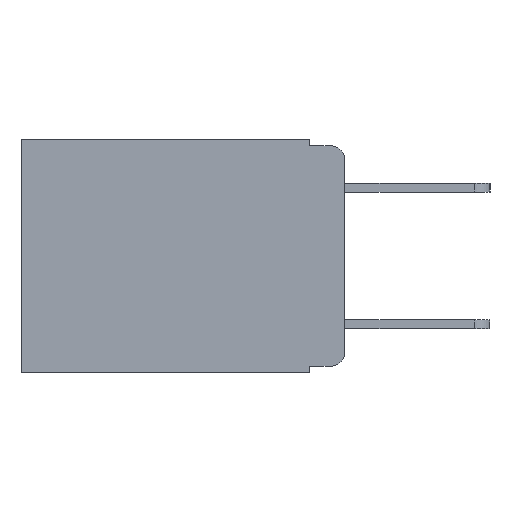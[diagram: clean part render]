
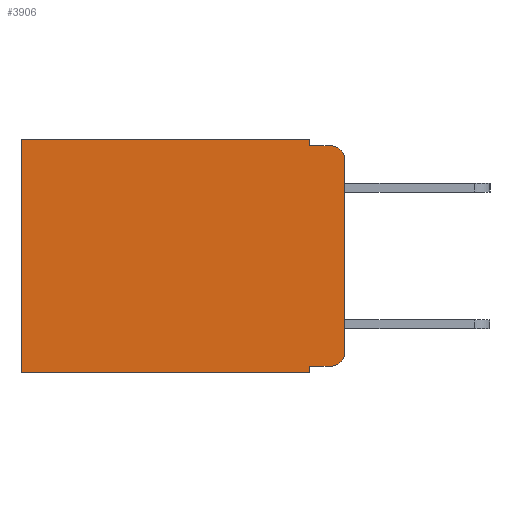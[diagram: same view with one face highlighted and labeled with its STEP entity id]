
A CAD part, left-side view. The second image highlights one B-rep face of the part: STEP entity #3906.
In plain terms, the highlighted planar face has unit normal (-1, 0, 0).
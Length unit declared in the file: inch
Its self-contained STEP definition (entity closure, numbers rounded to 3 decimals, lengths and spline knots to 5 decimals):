
#82 = CARTESIAN_POINT ( 'NONE',  ( 0.298, 0., -0.343 ) ) ;
#286 = CARTESIAN_POINT ( 'NONE',  ( 0.298, 0., 0. ) ) ;
#408 = AXIS2_PLACEMENT_3D ( 'NONE', #286, #2513, #8446 ) ;
#623 = CIRCLE ( 'NONE', #1907, 0.02 ) ;
#673 = LINE ( 'NONE', #2784, #7673 ) ;
#875 = CARTESIAN_POINT ( 'NONE',  ( 0.298, 0., 0. ) ) ;
#1018 = CARTESIAN_POINT ( 'NONE',  ( 0.298, 0., -0.313 ) ) ;
#1163 = LINE ( 'NONE', #875, #3454 ) ;
#1199 = EDGE_LOOP ( 'NONE', ( #7151, #10430, #8244, #7277, #4624, #6740, #10319, #8763, #6346, #9999 ) ) ;
#1327 = CARTESIAN_POINT ( 'NONE',  ( 0.298, 0., -0.03 ) ) ;
#1535 = VERTEX_POINT ( 'NONE', #8082 ) ;
#1851 = LINE ( 'NONE', #7398, #3890 ) ;
#1907 = AXIS2_PLACEMENT_3D ( 'NONE', #8008, #7997, #8992 ) ;
#2080 = CARTESIAN_POINT ( 'NONE',  ( 0.298, 0.051, -0.333 ) ) ;
#2082 = DIRECTION ( 'NONE',  ( 0., 0., -1. ) ) ;
#2168 = VERTEX_POINT ( 'NONE', #8883 ) ;
#2513 = DIRECTION ( 'NONE',  ( 1., 0., 0. ) ) ;
#2743 = CARTESIAN_POINT ( 'NONE',  ( 0.298, 0.02, -0.01 ) ) ;
#2784 = CARTESIAN_POINT ( 'NONE',  ( 0.298, 0.473, 0. ) ) ;
#2931 = VECTOR ( 'NONE', #10050, 39.37008 ) ;
#3118 = DIRECTION ( 'NONE',  ( 0., 0., -1. ) ) ;
#3124 = CARTESIAN_POINT ( 'NONE',  ( 0.298, 0.051, 0. ) ) ;
#3155 = CARTESIAN_POINT ( 'NONE',  ( 0.298, 0.051, 0. ) ) ;
#3364 = EDGE_CURVE ( 'NONE', #9633, #1535, #4097, .T. ) ;
#3365 = CIRCLE ( 'NONE', #4698, 0.02 ) ;
#3454 = VECTOR ( 'NONE', #5291, 39.37008 ) ;
#3890 = VECTOR ( 'NONE', #7408, 39.37008 ) ;
#3906 = ADVANCED_FACE ( 'NONE', ( #4807 ), #8005, .F. ) ;
#3939 = CARTESIAN_POINT ( 'NONE',  ( 0.298, 0.473, 0. ) ) ;
#3968 = VERTEX_POINT ( 'NONE', #2743 ) ;
#4042 = VERTEX_POINT ( 'NONE', #3124 ) ;
#4097 = LINE ( 'NONE', #82, #6246 ) ;
#4111 = DIRECTION ( 'NONE',  ( 0., 0., -1. ) ) ;
#4211 = DIRECTION ( 'NONE',  ( 0., 0., -1. ) ) ;
#4363 = EDGE_CURVE ( 'NONE', #5120, #5538, #3365, .T. ) ;
#4473 = EDGE_CURVE ( 'NONE', #2168, #5120, #8553, .T. ) ;
#4617 = EDGE_CURVE ( 'NONE', #2168, #9633, #9117, .T. ) ;
#4624 = ORIENTED_EDGE ( 'NONE', *, *, #6464, .T. ) ;
#4626 = DIRECTION ( 'NONE',  ( 0., 1., 0. ) ) ;
#4658 = CARTESIAN_POINT ( 'NONE',  ( 0.298, 0.051, -0.01 ) ) ;
#4698 = AXIS2_PLACEMENT_3D ( 'NONE', #10619, #10212, #4111 ) ;
#4703 = EDGE_CURVE ( 'NONE', #6406, #1535, #673, .T. ) ;
#4765 = DIRECTION ( 'NONE',  ( 0., -1., 0. ) ) ;
#4787 = EDGE_CURVE ( 'NONE', #4042, #5731, #10250, .T. ) ;
#4807 = FACE_OUTER_BOUND ( 'NONE', #1199, .T. ) ;
#5120 = VERTEX_POINT ( 'NONE', #8512 ) ;
#5291 = DIRECTION ( 'NONE',  ( 0., 0., -1. ) ) ;
#5335 = LINE ( 'NONE', #10032, #2931 ) ;
#5538 = VERTEX_POINT ( 'NONE', #1018 ) ;
#5731 = VERTEX_POINT ( 'NONE', #4658 ) ;
#6099 = EDGE_CURVE ( 'NONE', #5731, #3968, #5335, .T. ) ;
#6115 = EDGE_CURVE ( 'NONE', #10689, #3968, #623, .T. ) ;
#6246 = VECTOR ( 'NONE', #4626, 39.37008 ) ;
#6346 = ORIENTED_EDGE ( 'NONE', *, *, #4473, .T. ) ;
#6383 = VECTOR ( 'NONE', #4765, 39.37008 ) ;
#6406 = VERTEX_POINT ( 'NONE', #3939 ) ;
#6464 = EDGE_CURVE ( 'NONE', #4042, #6406, #1851, .T. ) ;
#6661 = VECTOR ( 'NONE', #2082, 39.37008 ) ;
#6671 = EDGE_CURVE ( 'NONE', #10689, #5538, #1163, .T. ) ;
#6740 = ORIENTED_EDGE ( 'NONE', *, *, #4703, .T. ) ;
#7151 = ORIENTED_EDGE ( 'NONE', *, *, #6671, .F. ) ;
#7277 = ORIENTED_EDGE ( 'NONE', *, *, #4787, .F. ) ;
#7398 = CARTESIAN_POINT ( 'NONE',  ( 0.298, 0., 0. ) ) ;
#7399 = CARTESIAN_POINT ( 'NONE',  ( 0.298, 0.051, 0. ) ) ;
#7408 = DIRECTION ( 'NONE',  ( 0., 1., 0. ) ) ;
#7673 = VECTOR ( 'NONE', #4211, 39.37008 ) ;
#7997 = DIRECTION ( 'NONE',  ( -1., 0., 0. ) ) ;
#8005 = PLANE ( 'NONE',  #408 ) ;
#8008 = CARTESIAN_POINT ( 'NONE',  ( 0.298, 0.02, -0.03 ) ) ;
#8082 = CARTESIAN_POINT ( 'NONE',  ( 0.298, 0.473, -0.343 ) ) ;
#8244 = ORIENTED_EDGE ( 'NONE', *, *, #6099, .F. ) ;
#8446 = DIRECTION ( 'NONE',  ( 0., 0., -1. ) ) ;
#8512 = CARTESIAN_POINT ( 'NONE',  ( 0.298, 0.02, -0.333 ) ) ;
#8553 = LINE ( 'NONE', #2080, #6383 ) ;
#8763 = ORIENTED_EDGE ( 'NONE', *, *, #4617, .F. ) ;
#8883 = CARTESIAN_POINT ( 'NONE',  ( 0.298, 0.051, -0.333 ) ) ;
#8901 = VECTOR ( 'NONE', #3118, 39.37008 ) ;
#8992 = DIRECTION ( 'NONE',  ( 0., 0., -1. ) ) ;
#9075 = CARTESIAN_POINT ( 'NONE',  ( 0.298, 0.051, -0.343 ) ) ;
#9117 = LINE ( 'NONE', #3155, #8901 ) ;
#9633 = VERTEX_POINT ( 'NONE', #9075 ) ;
#9999 = ORIENTED_EDGE ( 'NONE', *, *, #4363, .T. ) ;
#10032 = CARTESIAN_POINT ( 'NONE',  ( 0.298, 0.051, -0.01 ) ) ;
#10050 = DIRECTION ( 'NONE',  ( 0., -1., 0. ) ) ;
#10212 = DIRECTION ( 'NONE',  ( -1., 0., 0. ) ) ;
#10250 = LINE ( 'NONE', #7399, #6661 ) ;
#10319 = ORIENTED_EDGE ( 'NONE', *, *, #3364, .F. ) ;
#10430 = ORIENTED_EDGE ( 'NONE', *, *, #6115, .T. ) ;
#10619 = CARTESIAN_POINT ( 'NONE',  ( 0.298, 0.02, -0.313 ) ) ;
#10689 = VERTEX_POINT ( 'NONE', #1327 ) ;
